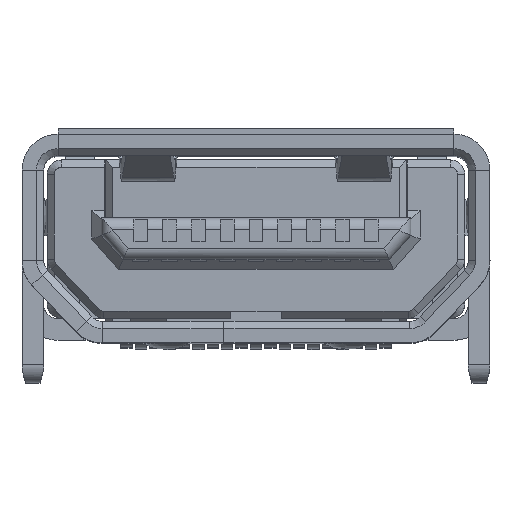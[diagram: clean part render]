
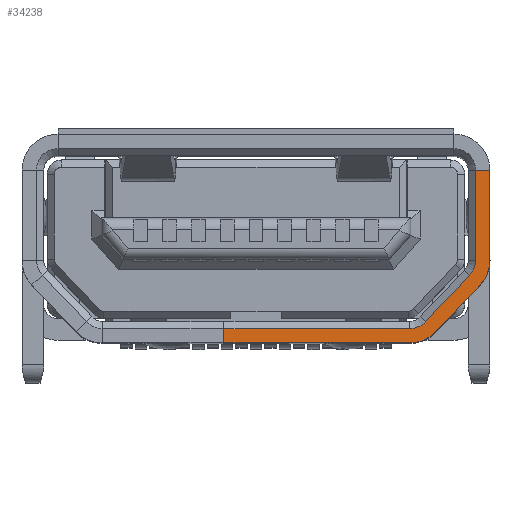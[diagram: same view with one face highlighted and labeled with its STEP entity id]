
A CAD part, top view. The second image highlights one B-rep face of the part: STEP entity #34238.
In plain terms, the highlighted planar face has unit normal (0, 0, 1).
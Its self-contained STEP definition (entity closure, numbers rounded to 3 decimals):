
#657 = EDGE_CURVE ( 'NONE', #63218, #57879, #31169, .T. ) ;
#912 = ORIENTED_EDGE ( 'NONE', *, *, #57202, .F. ) ;
#941 = VERTEX_POINT ( 'NONE', #20378 ) ;
#1725 = CARTESIAN_POINT ( 'NONE',  ( 2.75, -1.75, 0. ) ) ;
#3506 = CARTESIAN_POINT ( 'NONE',  ( 3.05, -0.5, 0. ) ) ;
#4649 = CARTESIAN_POINT ( 'NONE',  ( 3.25, -1.882, 0. ) ) ;
#5266 = CARTESIAN_POINT ( 'NONE',  ( 2.805, -2.419, 0. ) ) ;
#6608 = FACE_OUTER_BOUND ( 'NONE', #56517, .T. ) ;
#8394 = VECTOR ( 'NONE', #35032, 1000. ) ;
#8815 = DIRECTION ( 'NONE',  ( 1., 0., 0. ) ) ;
#9329 = LINE ( 'NONE', #4649, #8394 ) ;
#9638 = CIRCLE ( 'NONE', #27694, 0.3 ) ;
#10074 = CARTESIAN_POINT ( 'NONE',  ( 0.845, -2.9, 0. ) ) ;
#10694 = B_SPLINE_CURVE_WITH_KNOTS ( 'NONE', 3,
 ( #17623, #60056, #29624, #24628 ),
 .UNSPECIFIED., .F., .F.,
 ( 4, 4 ),
 ( 0., 0. ),
 .UNSPECIFIED. ) ;
#11433 = AXIS2_PLACEMENT_3D ( 'NONE', #52728, #63699, #12582 ) ;
#11838 = EDGE_CURVE ( 'NONE', #51164, #36056, #51134, .T. ) ;
#12582 = DIRECTION ( 'NONE',  ( -1., 0., 0. ) ) ;
#13373 = CARTESIAN_POINT ( 'NONE',  ( 3.05, -0.5, 0. ) ) ;
#15034 = LINE ( 'NONE', #10074, #25991 ) ;
#15403 = DIRECTION ( 'NONE',  ( 1., 0., 0. ) ) ;
#15646 = DIRECTION ( 'NONE',  ( 0., 0., 1. ) ) ;
#16790 = EDGE_CURVE ( 'NONE', #24591, #941, #22003, .T. ) ;
#17218 = CARTESIAN_POINT ( 'NONE',  ( 2.352, -2.606, 0. ) ) ;
#17623 = CARTESIAN_POINT ( 'NONE',  ( 3.113, -2.094, 0. ) ) ;
#17629 = AXIS2_PLACEMENT_3D ( 'NONE', #34202, #38200, #8815 ) ;
#18364 = CARTESIAN_POINT ( 'NONE',  ( 3.183, -0.5, 0. ) ) ;
#18589 = EDGE_CURVE ( 'NONE', #60683, #51164, #39087, .T. ) ;
#19961 = CARTESIAN_POINT ( 'NONE',  ( 2.134, -2.4, 0. ) ) ;
#20212 = CARTESIAN_POINT ( 'NONE',  ( -0.445, -2.9, 0. ) ) ;
#20370 = CARTESIAN_POINT ( 'NONE',  ( 3.05, -0.475, 0. ) ) ;
#20378 = CARTESIAN_POINT ( 'NONE',  ( 2.497, -2.744, 0. ) ) ;
#22003 = CIRCLE ( 'NONE', #17629, 0.5 ) ;
#22511 = DIRECTION ( 'NONE',  ( 0.688, 0.726, 0. ) ) ;
#24591 = VERTEX_POINT ( 'NONE', #64723 ) ;
#24628 = CARTESIAN_POINT ( 'NONE',  ( 3.25, -1.75, 0. ) ) ;
#24705 = CARTESIAN_POINT ( 'NONE',  ( 3.25, -0.5, 0. ) ) ;
#25499 = CARTESIAN_POINT ( 'NONE',  ( 0.845, -2.7, 0. ) ) ;
#25991 = VECTOR ( 'NONE', #30091, 1000. ) ;
#27512 = CARTESIAN_POINT ( 'NONE',  ( 2.66, -2.282, 0. ) ) ;
#27694 = AXIS2_PLACEMENT_3D ( 'NONE', #1725, #15646, #36079 ) ;
#28491 = CARTESIAN_POINT ( 'NONE',  ( 3.25, -1.75, 0. ) ) ;
#28825 = ORIENTED_EDGE ( 'NONE', *, *, #18589, .T. ) ;
#29610 = EDGE_CURVE ( 'NONE', #40745, #24591, #15034, .T. ) ;
#29624 = CARTESIAN_POINT ( 'NONE',  ( 3.25, -1.878, 0. ) ) ;
#29701 = AXIS2_PLACEMENT_3D ( 'NONE', #19961, #39707, #50073 ) ;
#29980 = CARTESIAN_POINT ( 'NONE',  ( 2.968, -1.957, 0. ) ) ;
#30091 = DIRECTION ( 'NONE',  ( 1., 0., 0. ) ) ;
#30289 = EDGE_CURVE ( 'NONE', #36125, #41446, #10694, .T. ) ;
#30585 = VECTOR ( 'NONE', #61038, 1000. ) ;
#31169 = LINE ( 'NONE', #25499, #55150 ) ;
#34202 = CARTESIAN_POINT ( 'NONE',  ( 2.134, -2.4, 0. ) ) ;
#34238 = ADVANCED_FACE ( 'NONE', ( #6608 ), #57726, .T. ) ;
#35032 = DIRECTION ( 'NONE',  ( 0., -1., 0. ) ) ;
#35119 = DIRECTION ( 'NONE',  ( 0., -1., 0. ) ) ;
#36056 = VERTEX_POINT ( 'NONE', #45588 ) ;
#36079 = DIRECTION ( 'NONE',  ( 1., 0., 0. ) ) ;
#36125 = VERTEX_POINT ( 'NONE', #45919 ) ;
#36570 = VECTOR ( 'NONE', #22511, 1000. ) ;
#36690 = ORIENTED_EDGE ( 'NONE', *, *, #657, .F. ) ;
#38200 = DIRECTION ( 'NONE',  ( 0., 0., 1. ) ) ;
#38503 = ORIENTED_EDGE ( 'NONE', *, *, #40049, .F. ) ;
#39087 = B_SPLINE_CURVE_WITH_KNOTS ( 'NONE', 3,
 ( #64185, #18364, #59176, #13373 ),
 .UNSPECIFIED., .F., .F.,
 ( 4, 4 ),
 ( 0., 1. ),
 .UNSPECIFIED. ) ;
#39099 = CARTESIAN_POINT ( 'NONE',  ( -0.445, -2.75, 0. ) ) ;
#39707 = DIRECTION ( 'NONE',  ( 0., 0., 1. ) ) ;
#40049 = EDGE_CURVE ( 'NONE', #60818, #56123, #62625, .T. ) ;
#40745 = VERTEX_POINT ( 'NONE', #20212 ) ;
#41446 = VERTEX_POINT ( 'NONE', #28491 ) ;
#41642 = LINE ( 'NONE', #5266, #30585 ) ;
#43849 = EDGE_CURVE ( 'NONE', #36125, #941, #41642, .T. ) ;
#45141 = CARTESIAN_POINT ( 'NONE',  ( 2.134, -2.7, 0. ) ) ;
#45588 = CARTESIAN_POINT ( 'NONE',  ( 3.05, -1.75, 0. ) ) ;
#45919 = CARTESIAN_POINT ( 'NONE',  ( 3.113, -2.094, 0. ) ) ;
#46790 = VECTOR ( 'NONE', #59474, 1000. ) ;
#48494 = EDGE_CURVE ( 'NONE', #63218, #40745, #64474, .T. ) ;
#49582 = ORIENTED_EDGE ( 'NONE', *, *, #48494, .T. ) ;
#49623 = ORIENTED_EDGE ( 'NONE', *, *, #16790, .T. ) ;
#50073 = DIRECTION ( 'NONE',  ( 1., 0., 0. ) ) ;
#50513 = EDGE_CURVE ( 'NONE', #56123, #36056, #9638, .T. ) ;
#51134 = LINE ( 'NONE', #20370, #55384 ) ;
#51164 = VERTEX_POINT ( 'NONE', #3506 ) ;
#51923 = ORIENTED_EDGE ( 'NONE', *, *, #43849, .F. ) ;
#51994 = CARTESIAN_POINT ( 'NONE',  ( -0.445, -2.7, 0. ) ) ;
#52104 = ORIENTED_EDGE ( 'NONE', *, *, #30289, .T. ) ;
#52728 = CARTESIAN_POINT ( 'NONE',  ( 2.186, -2.687, 0. ) ) ;
#55150 = VECTOR ( 'NONE', #15403, 1000. ) ;
#55384 = VECTOR ( 'NONE', #35119, 1000. ) ;
#56123 = VERTEX_POINT ( 'NONE', #29980 ) ;
#56517 = EDGE_LOOP ( 'NONE', ( #65670, #49623, #51923, #52104, #64796, #28825, #57597, #60629, #38503, #912, #36690, #49582 ) ) ;
#57172 = EDGE_CURVE ( 'NONE', #60683, #41446, #9329, .T. ) ;
#57202 = EDGE_CURVE ( 'NONE', #57879, #60818, #59613, .T. ) ;
#57597 = ORIENTED_EDGE ( 'NONE', *, *, #11838, .T. ) ;
#57726 = PLANE ( 'NONE',  #11433 ) ;
#57879 = VERTEX_POINT ( 'NONE', #45141 ) ;
#59176 = CARTESIAN_POINT ( 'NONE',  ( 3.117, -0.5, 0. ) ) ;
#59474 = DIRECTION ( 'NONE',  ( 0., -1., 0. ) ) ;
#59613 = CIRCLE ( 'NONE', #29701, 0.3 ) ;
#60056 = CARTESIAN_POINT ( 'NONE',  ( 3.201, -2.002, 0. ) ) ;
#60629 = ORIENTED_EDGE ( 'NONE', *, *, #50513, .F. ) ;
#60683 = VERTEX_POINT ( 'NONE', #24705 ) ;
#60818 = VERTEX_POINT ( 'NONE', #17218 ) ;
#61038 = DIRECTION ( 'NONE',  ( -0.688, -0.726, 0. ) ) ;
#62625 = LINE ( 'NONE', #27512, #36570 ) ;
#63218 = VERTEX_POINT ( 'NONE', #51994 ) ;
#63699 = DIRECTION ( 'NONE',  ( 0., 0., 1. ) ) ;
#64185 = CARTESIAN_POINT ( 'NONE',  ( 3.25, -0.5, 0. ) ) ;
#64474 = LINE ( 'NONE', #39099, #46790 ) ;
#64723 = CARTESIAN_POINT ( 'NONE',  ( 2.134, -2.9, 0. ) ) ;
#64796 = ORIENTED_EDGE ( 'NONE', *, *, #57172, .F. ) ;
#65670 = ORIENTED_EDGE ( 'NONE', *, *, #29610, .T. ) ;
